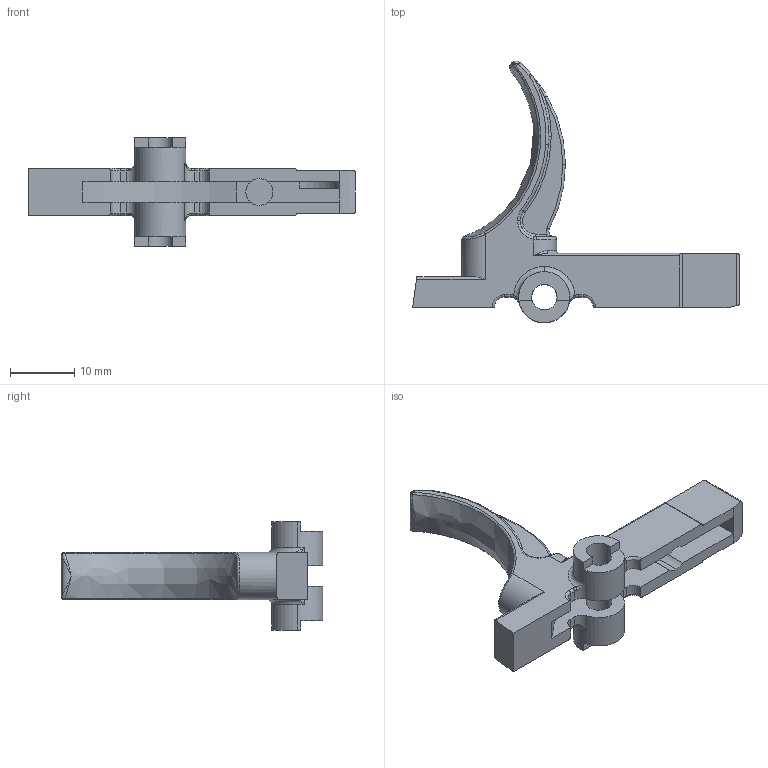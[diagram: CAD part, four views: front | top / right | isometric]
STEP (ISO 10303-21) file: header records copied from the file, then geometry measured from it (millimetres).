
FILE_DESCRIPTION (( 'STEP AP214' ), '1' );
FILE_NAME ('Trigger.step.step', '2019-12-18T03:08:59', ( '' ), ( '' ), 'SwSTEP 2.0', 'SolidWorks 2019', '' );
FILE_SCHEMA (( 'AUTOMOTIVE_DESIGN' ));
Length unit declared in the file: millimetre
Products named in the file (1): Trigger.step
Bounding box: 51.01 x 40.83 x 16.87 mm (x, y, z)
Volume: 3393.3 mm3; surface area: 3182.6 mm2
Topology: 1 solids, 1 shells, 172 faces, 451 edges, 267 vertices
Faces by surface type: cylinder 59, torus 42, plane 41, bspline 26, sphere 4
Entity records: 6897 total; most frequent: CARTESIAN_POINT 2750, DIRECTION 887, ORIENTED_EDGE 878, EDGE_CURVE 439, AXIS2_PLACEMENT_3D 367, VERTEX_POINT 267, CIRCLE 220, EDGE_LOOP 174
